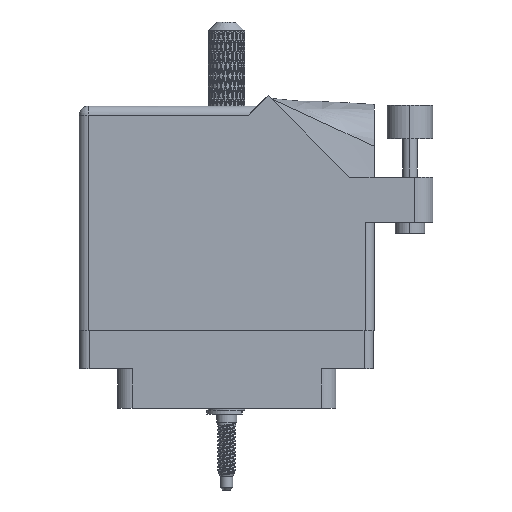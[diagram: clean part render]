
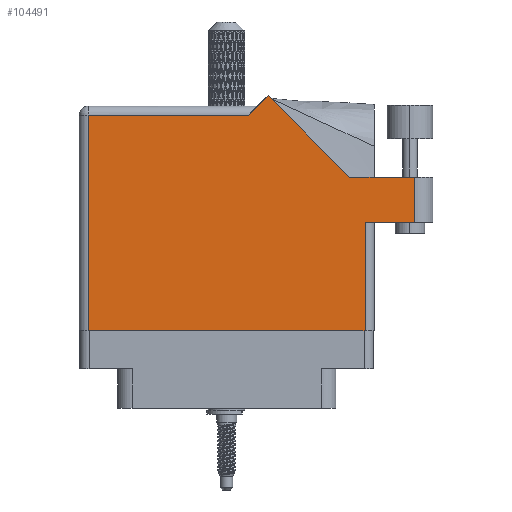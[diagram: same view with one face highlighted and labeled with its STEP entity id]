
A CAD part, front view. The second image highlights one B-rep face of the part: STEP entity #104491.
In plain terms, the highlighted face is planar.
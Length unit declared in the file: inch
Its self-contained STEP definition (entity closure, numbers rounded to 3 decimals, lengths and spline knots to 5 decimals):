
#7059 = DIRECTION ( 'NONE',  ( 0., 1., 0. ) ) ;
#10003 = CARTESIAN_POINT ( 'NONE',  ( 2.285, 1.044, 0. ) ) ;
#10345 = ORIENTED_EDGE ( 'NONE', *, *, #23338, .T. ) ;
#10734 = CARTESIAN_POINT ( 'NONE',  ( 2.285, 1.044, 0. ) ) ;
#11222 = ORIENTED_EDGE ( 'NONE', *, *, #45080, .T. ) ;
#11436 = CARTESIAN_POINT ( 'NONE',  ( 1.948, 0., 0. ) ) ;
#13709 = ORIENTED_EDGE ( 'NONE', *, *, #102119, .T. ) ;
#14141 = VECTOR ( 'NONE', #71364, 39.37008 ) ;
#15488 = ORIENTED_EDGE ( 'NONE', *, *, #32768, .T. ) ;
#16164 = CARTESIAN_POINT ( 'NONE',  ( 1.28771, 1.60071, 0. ) ) ;
#17589 = ORIENTED_EDGE ( 'NONE', *, *, #80575, .T. ) ;
#17787 = CARTESIAN_POINT ( 'NONE',  ( 2.285, 0.737, 0. ) ) ;
#20897 = CARTESIAN_POINT ( 'NONE',  ( 1.948, 0.737, 0. ) ) ;
#23338 = EDGE_CURVE ( 'NONE', #54849, #58567, #26760, .T. ) ;
#23746 = CARTESIAN_POINT ( 'NONE',  ( 1.84442, 1.044, 0. ) ) ;
#25938 = LINE ( 'NONE', #102362, #88000 ) ;
#26467 = VECTOR ( 'NONE', #73352, 39.37008 ) ;
#26760 = LINE ( 'NONE', #103108, #14141 ) ;
#27566 = AXIS2_PLACEMENT_3D ( 'NONE', #89615, #41154, #97709 ) ;
#29479 = CARTESIAN_POINT ( 'NONE',  ( 1.217, 1.53, 0. ) ) ;
#30690 = LINE ( 'NONE', #29479, #37007 ) ;
#30714 = VECTOR ( 'NONE', #87766, 39.37008 ) ;
#31672 = LINE ( 'NONE', #20897, #65910 ) ;
#31904 = DIRECTION ( 'NONE',  ( 0., -1., 0. ) ) ;
#32602 = EDGE_CURVE ( 'NONE', #59175, #86096, #25938, .T. ) ;
#32768 = EDGE_CURVE ( 'NONE', #34310, #66800, #99826, .T. ) ;
#33695 = VERTEX_POINT ( 'NONE', #36262 ) ;
#34310 = VERTEX_POINT ( 'NONE', #10734 ) ;
#34395 = DIRECTION ( 'NONE',  ( 0., 1., 0. ) ) ;
#36262 = CARTESIAN_POINT ( 'NONE',  ( 1.155, 1.468, 0. ) ) ;
#37007 = VECTOR ( 'NONE', #38623, 39.37008 ) ;
#37348 = CARTESIAN_POINT ( 'NONE',  ( 1.84442, 1.044, 0. ) ) ;
#37408 = LINE ( 'NONE', #64103, #77906 ) ;
#38536 = EDGE_LOOP ( 'NONE', ( #58690, #56606, #15488, #13709, #11222, #101607, #17589, #10345, #75924 ) ) ;
#38623 = DIRECTION ( 'NONE',  ( -0.707, -0.707, 0. ) ) ;
#41154 = DIRECTION ( 'NONE',  ( 0., 0., -1. ) ) ;
#45080 = EDGE_CURVE ( 'NONE', #55126, #33695, #30690, .T. ) ;
#45193 = DIRECTION ( 'NONE',  ( 1., 0., 0. ) ) ;
#47817 = CARTESIAN_POINT ( 'NONE',  ( 0.062, 1.468, 0. ) ) ;
#48165 = FACE_OUTER_BOUND ( 'NONE', #38536, .T. ) ;
#53381 = EDGE_CURVE ( 'NONE', #86096, #34310, #75257, .T. ) ;
#54849 = VERTEX_POINT ( 'NONE', #87429 ) ;
#55126 = VERTEX_POINT ( 'NONE', #16164 ) ;
#56057 = LINE ( 'NONE', #94528, #30714 ) ;
#56606 = ORIENTED_EDGE ( 'NONE', *, *, #53381, .T. ) ;
#57826 = VERTEX_POINT ( 'NONE', #47817 ) ;
#58567 = VERTEX_POINT ( 'NONE', #11436 ) ;
#58690 = ORIENTED_EDGE ( 'NONE', *, *, #32602, .T. ) ;
#59175 = VERTEX_POINT ( 'NONE', #102681 ) ;
#64103 = CARTESIAN_POINT ( 'NONE',  ( 0.062, 0., 0. ) ) ;
#65910 = VECTOR ( 'NONE', #7059, 39.37008 ) ;
#66800 = VERTEX_POINT ( 'NONE', #37348 ) ;
#71364 = DIRECTION ( 'NONE',  ( 1., 0., 0. ) ) ;
#72992 = CARTESIAN_POINT ( 'NONE',  ( 2.41, 1.044, 0. ) ) ;
#73352 = DIRECTION ( 'NONE',  ( -1., 0., 0. ) ) ;
#73449 = EDGE_CURVE ( 'NONE', #58567, #59175, #31672, .T. ) ;
#73476 = VECTOR ( 'NONE', #80351, 39.37008 ) ;
#75066 = PLANE ( 'NONE',  #27566 ) ;
#75257 = LINE ( 'NONE', #10003, #93066 ) ;
#75924 = ORIENTED_EDGE ( 'NONE', *, *, #73449, .T. ) ;
#77906 = VECTOR ( 'NONE', #31904, 39.37008 ) ;
#80351 = DIRECTION ( 'NONE',  ( -0.707, 0.707, 0. ) ) ;
#80575 = EDGE_CURVE ( 'NONE', #57826, #54849, #37408, .T. ) ;
#86096 = VERTEX_POINT ( 'NONE', #17787 ) ;
#87065 = EDGE_CURVE ( 'NONE', #33695, #57826, #56057, .T. ) ;
#87429 = CARTESIAN_POINT ( 'NONE',  ( 0.062, 0., 0. ) ) ;
#87766 = DIRECTION ( 'NONE',  ( -1., 0., 0. ) ) ;
#88000 = VECTOR ( 'NONE', #45193, 39.37008 ) ;
#89615 = CARTESIAN_POINT ( 'NONE',  ( 0., 1.53, 0. ) ) ;
#93066 = VECTOR ( 'NONE', #34395, 39.37008 ) ;
#94528 = CARTESIAN_POINT ( 'NONE',  ( 0., 1.468, 0. ) ) ;
#95005 = LINE ( 'NONE', #23746, #73476 ) ;
#97709 = DIRECTION ( 'NONE',  ( -1., 0., 0. ) ) ;
#99826 = LINE ( 'NONE', #72992, #26467 ) ;
#101607 = ORIENTED_EDGE ( 'NONE', *, *, #87065, .T. ) ;
#102119 = EDGE_CURVE ( 'NONE', #66800, #55126, #95005, .T. ) ;
#102362 = CARTESIAN_POINT ( 'NONE',  ( 2.01, 0.737, 0. ) ) ;
#102681 = CARTESIAN_POINT ( 'NONE',  ( 1.948, 0.737, 0. ) ) ;
#103108 = CARTESIAN_POINT ( 'NONE',  ( 0., 0., 0. ) ) ;
#104491 = ADVANCED_FACE ( 'NONE', ( #48165 ), #75066, .F. ) ;
